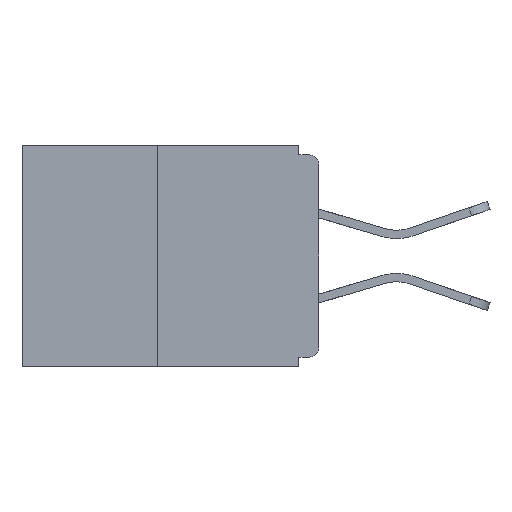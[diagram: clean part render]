
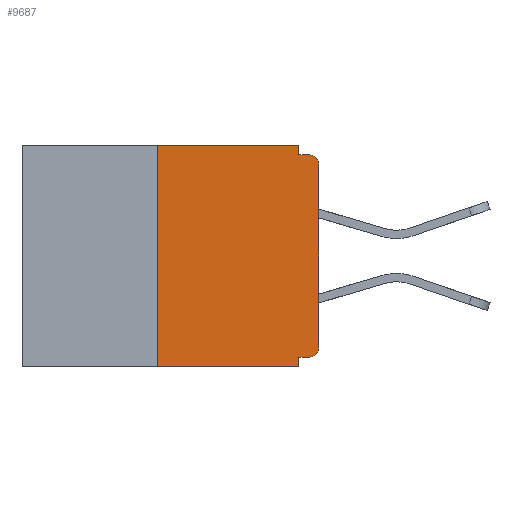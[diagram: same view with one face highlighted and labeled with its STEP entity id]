
A CAD part, left-side view. The second image highlights one B-rep face of the part: STEP entity #9687.
In plain terms, the highlighted planar face has unit normal (-1, 0, 0).
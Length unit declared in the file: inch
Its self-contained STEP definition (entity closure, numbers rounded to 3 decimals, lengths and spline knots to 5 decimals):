
#49 = CARTESIAN_POINT ( 'NONE',  ( 0., 0.031, 0. ) ) ;
#100 = EDGE_CURVE ( 'NONE', #7858, #914, #5536, .T. ) ;
#141 = PLANE ( 'NONE',  #6711 ) ;
#273 = VERTEX_POINT ( 'NONE', #8331 ) ;
#659 = EDGE_CURVE ( 'NONE', #2362, #273, #7966, .T. ) ;
#693 = VECTOR ( 'NONE', #10122, 39.37008 ) ;
#781 = FACE_OUTER_BOUND ( 'NONE', #6233, .T. ) ;
#914 = VERTEX_POINT ( 'NONE', #3351 ) ;
#1537 = DIRECTION ( 'NONE',  ( 0., -1., 0. ) ) ;
#1675 = VECTOR ( 'NONE', #3575, 39.37008 ) ;
#1683 = DIRECTION ( 'NONE',  ( 0., 0., -1. ) ) ;
#2041 = LINE ( 'NONE', #6475, #10148 ) ;
#2205 = LINE ( 'NONE', #5452, #13231 ) ;
#2230 = CARTESIAN_POINT ( 'NONE',  ( 0., 0.015, -0.313 ) ) ;
#2234 = AXIS2_PLACEMENT_3D ( 'NONE', #2639, #7814, #1683 ) ;
#2362 = VERTEX_POINT ( 'NONE', #11635 ) ;
#2453 = VERTEX_POINT ( 'NONE', #12815 ) ;
#2639 = CARTESIAN_POINT ( 'NONE',  ( 0., 0.015, -0.03 ) ) ;
#2691 = DIRECTION ( 'NONE',  ( 0., -1., 0. ) ) ;
#2719 = ORIENTED_EDGE ( 'NONE', *, *, #8049, .F. ) ;
#2812 = ORIENTED_EDGE ( 'NONE', *, *, #6286, .T. ) ;
#3103 = ORIENTED_EDGE ( 'NONE', *, *, #8100, .T. ) ;
#3104 = EDGE_CURVE ( 'NONE', #914, #3170, #5071, .T. ) ;
#3157 = VERTEX_POINT ( 'NONE', #4826 ) ;
#3170 = VERTEX_POINT ( 'NONE', #12106 ) ;
#3351 = CARTESIAN_POINT ( 'NONE',  ( 0., 0.031, -0.328 ) ) ;
#3575 = DIRECTION ( 'NONE',  ( 0., 0., -1. ) ) ;
#3719 = CARTESIAN_POINT ( 'NONE',  ( 0., 0., -0.313 ) ) ;
#4225 = DIRECTION ( 'NONE',  ( -1., 0., 0. ) ) ;
#4292 = LINE ( 'NONE', #49, #12245 ) ;
#4658 = CARTESIAN_POINT ( 'NONE',  ( 0., 0.46, 0. ) ) ;
#4726 = LINE ( 'NONE', #4658, #11231 ) ;
#4826 = CARTESIAN_POINT ( 'NONE',  ( 0., 0.031, 0. ) ) ;
#5071 = LINE ( 'NONE', #5824, #1675 ) ;
#5195 = DIRECTION ( 'NONE',  ( 0., 0., -1. ) ) ;
#5452 = CARTESIAN_POINT ( 'NONE',  ( 0., 0., -0.015 ) ) ;
#5536 = LINE ( 'NONE', #8987, #11545 ) ;
#5809 = CARTESIAN_POINT ( 'NONE',  ( 0., 0.25, 0. ) ) ;
#5824 = CARTESIAN_POINT ( 'NONE',  ( 0., 0.031, -0.343 ) ) ;
#6233 = EDGE_LOOP ( 'NONE', ( #12601, #7604, #2812, #10354, #8618, #8163, #3103, #9314, #2719, #13024 ) ) ;
#6286 = EDGE_CURVE ( 'NONE', #2362, #3170, #11491, .T. ) ;
#6475 = CARTESIAN_POINT ( 'NONE',  ( 0., 0., 0. ) ) ;
#6667 = EDGE_CURVE ( 'NONE', #7858, #8377, #7925, .T. ) ;
#6711 = AXIS2_PLACEMENT_3D ( 'NONE', #8597, #10729, #11775 ) ;
#6816 = CARTESIAN_POINT ( 'NONE',  ( 0., 0., -0.03 ) ) ;
#7264 = DIRECTION ( 'NONE',  ( 0., 0., -1. ) ) ;
#7497 = VERTEX_POINT ( 'NONE', #6816 ) ;
#7604 = ORIENTED_EDGE ( 'NONE', *, *, #659, .F. ) ;
#7814 = DIRECTION ( 'NONE',  ( -1., 0., 0. ) ) ;
#7858 = VERTEX_POINT ( 'NONE', #13318 ) ;
#7925 = CIRCLE ( 'NONE', #11369, 0.015 ) ;
#7966 = LINE ( 'NONE', #5809, #693 ) ;
#8049 = EDGE_CURVE ( 'NONE', #2453, #10724, #2205, .T. ) ;
#8100 = EDGE_CURVE ( 'NONE', #8377, #7497, #2041, .T. ) ;
#8163 = ORIENTED_EDGE ( 'NONE', *, *, #6667, .T. ) ;
#8331 = CARTESIAN_POINT ( 'NONE',  ( 0., 0.25, 0. ) ) ;
#8377 = VERTEX_POINT ( 'NONE', #3719 ) ;
#8597 = CARTESIAN_POINT ( 'NONE',  ( 0., 0.46, 0. ) ) ;
#8618 = ORIENTED_EDGE ( 'NONE', *, *, #100, .F. ) ;
#8747 = DIRECTION ( 'NONE',  ( 0., 0., 1. ) ) ;
#8987 = CARTESIAN_POINT ( 'NONE',  ( 0., 0., -0.328 ) ) ;
#9314 = ORIENTED_EDGE ( 'NONE', *, *, #12676, .T. ) ;
#9638 = DIRECTION ( 'NONE',  ( 0., -1., 0. ) ) ;
#9687 = ADVANCED_FACE ( 'NONE', ( #781 ), #141, .F. ) ;
#9987 = DIRECTION ( 'NONE',  ( 0., 1., 0. ) ) ;
#10067 = CIRCLE ( 'NONE', #2234, 0.015 ) ;
#10122 = DIRECTION ( 'NONE',  ( 0., 0., 1. ) ) ;
#10148 = VECTOR ( 'NONE', #8747, 39.37008 ) ;
#10354 = ORIENTED_EDGE ( 'NONE', *, *, #3104, .F. ) ;
#10724 = VERTEX_POINT ( 'NONE', #11122 ) ;
#10729 = DIRECTION ( 'NONE',  ( 1., 0., 0. ) ) ;
#10919 = EDGE_CURVE ( 'NONE', #3157, #2453, #4292, .T. ) ;
#11122 = CARTESIAN_POINT ( 'NONE',  ( 0., 0.015, -0.015 ) ) ;
#11231 = VECTOR ( 'NONE', #2691, 39.37008 ) ;
#11369 = AXIS2_PLACEMENT_3D ( 'NONE', #2230, #4225, #7264 ) ;
#11491 = LINE ( 'NONE', #11958, #12952 ) ;
#11545 = VECTOR ( 'NONE', #9987, 39.37008 ) ;
#11620 = EDGE_CURVE ( 'NONE', #273, #3157, #4726, .T. ) ;
#11635 = CARTESIAN_POINT ( 'NONE',  ( 0., 0.25, -0.343 ) ) ;
#11775 = DIRECTION ( 'NONE',  ( 0., 0., -1. ) ) ;
#11958 = CARTESIAN_POINT ( 'NONE',  ( 0., 0.46, -0.343 ) ) ;
#12106 = CARTESIAN_POINT ( 'NONE',  ( 0., 0.031, -0.343 ) ) ;
#12245 = VECTOR ( 'NONE', #5195, 39.37008 ) ;
#12601 = ORIENTED_EDGE ( 'NONE', *, *, #11620, .F. ) ;
#12676 = EDGE_CURVE ( 'NONE', #7497, #10724, #10067, .T. ) ;
#12815 = CARTESIAN_POINT ( 'NONE',  ( 0., 0.031, -0.015 ) ) ;
#12952 = VECTOR ( 'NONE', #1537, 39.37008 ) ;
#13024 = ORIENTED_EDGE ( 'NONE', *, *, #10919, .F. ) ;
#13231 = VECTOR ( 'NONE', #9638, 39.37008 ) ;
#13318 = CARTESIAN_POINT ( 'NONE',  ( 0., 0.015, -0.328 ) ) ;
